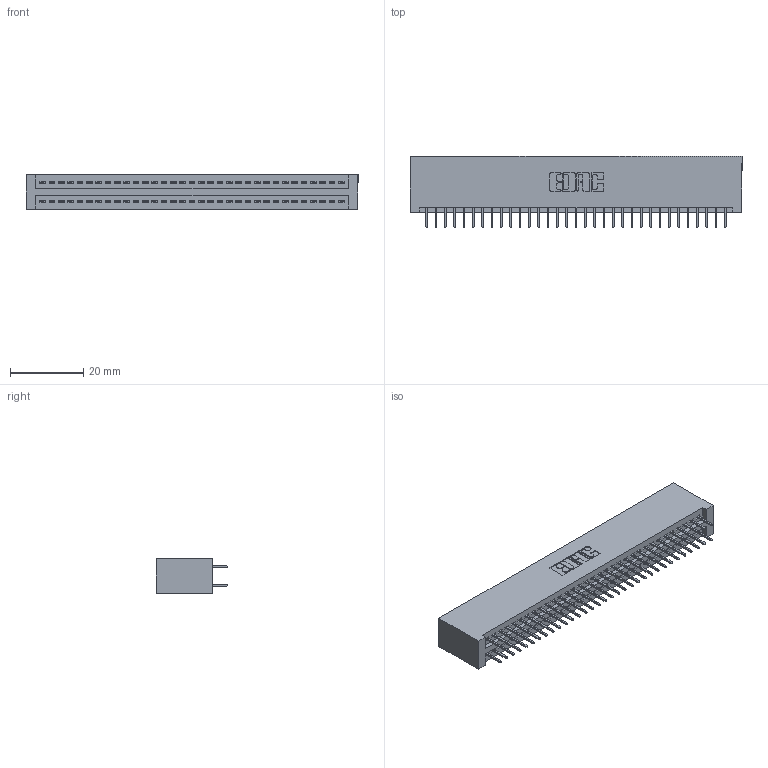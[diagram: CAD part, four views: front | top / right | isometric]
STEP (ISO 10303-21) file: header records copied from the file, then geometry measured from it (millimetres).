
FILE_DESCRIPTION (( 'STEP AP203' ), '1' );
FILE_NAME ('345-066-524-201.STEP', '2019-10-30T16:40:49', ( '' ), ( '' ), 'SwSTEP 2.0', 'SolidWorks 2016', '' );
FILE_SCHEMA (( 'CONFIG_CONTROL_DESIGN' ));
Length unit declared in the file: inch
Products named in the file (3): 345-066-524-201; 345 Part_No Mounting Lugs; 345-292-001_345-293-124
Assembly tree (67 placements, depth 2):
  345-066-524-201
    345 Part_No Mounting Lugs
    345-292-001_345-293-124  x66
Bounding box: 90.42 x 19.35 x 9.4 mm (x, y, z)
Volume: 9216.4 mm3; surface area: 13488.6 mm2
Topology: 67 solids, 67 shells, 3682 faces, 10415 edges, 6678 vertices
Faces by surface type: plane 2650, cylinder 1032
Entity records: 26901 total; most frequent: CARTESIAN_POINT 4516, ORIENTED_EDGE 4450, DIRECTION 3989, EDGE_CURVE 2225, VECTOR 1973, LINE 1973, VERTEX_POINT 1478, AXIS2_PLACEMENT_3D 1008
